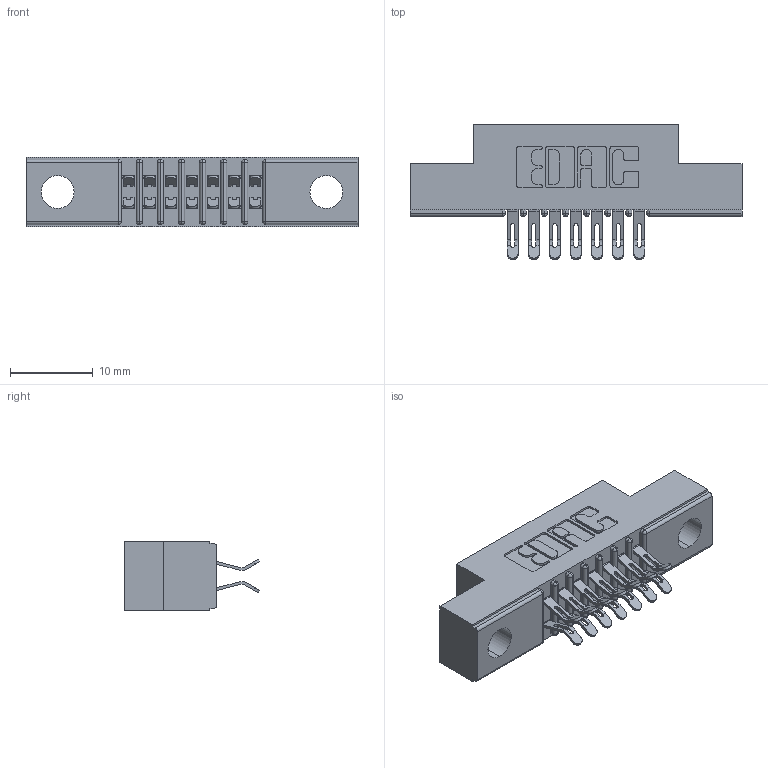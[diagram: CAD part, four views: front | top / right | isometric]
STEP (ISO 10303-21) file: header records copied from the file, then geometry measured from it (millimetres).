
FILE_DESCRIPTION (( 'STEP AP203' ), '1' );
FILE_NAME ('341-014-555-204.STEP', '2018-08-06T15:18:20', ( '' ), ( '' ), 'SwSTEP 2.0', 'SolidWorks 2016', '' );
FILE_SCHEMA (( 'CONFIG_CONTROL_DESIGN' ));
Length unit declared in the file: inch
Products named in the file (3): 341 Part_.156 (3.96) Dia Mounting Holes; 341-292-001_341-292-155; 341-014-555-204
Assembly tree (15 placements, depth 2):
  341-014-555-204
    341 Part_.156 (3.96) Dia Mounting Holes
    341-292-001_341-292-155  x14
Bounding box: 40.01 x 16.31 x 8.38 mm (x, y, z)
Volume: 2230.3 mm3; surface area: 3749.5 mm2
Topology: 15 solids, 15 shells, 1222 faces, 3621 edges, 2358 vertices
Faces by surface type: plane 670, cylinder 524, sphere 16, torus 12
Entity records: 14022 total; most frequent: CARTESIAN_POINT 2353, ORIENTED_EDGE 2322, DIRECTION 2291, EDGE_CURVE 1161, LINE 891, VECTOR 891, VERTEX_POINT 746, AXIS2_PLACEMENT_3D 700
